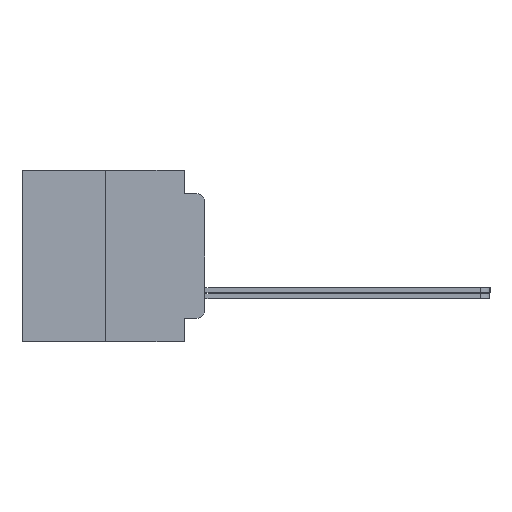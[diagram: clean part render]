
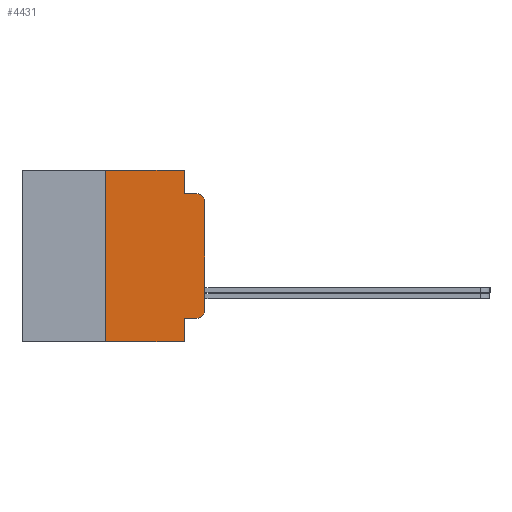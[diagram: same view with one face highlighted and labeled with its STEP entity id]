
A CAD part, left-side view. The second image highlights one B-rep face of the part: STEP entity #4431.
In plain terms, the highlighted planar face has unit normal (-1, 0, 0).
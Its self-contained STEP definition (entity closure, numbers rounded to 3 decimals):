
#132 = VECTOR ( 'NONE', #7905, 1000. ) ;
#256 = DIRECTION ( 'NONE',  ( -1., 0., 0. ) ) ;
#378 = CARTESIAN_POINT ( 'NONE',  ( -75.603, 6.35, -5.486 ) ) ;
#1163 = PLANE ( 'NONE',  #27982 ) ;
#1304 = EDGE_CURVE ( 'NONE', #25499, #4151, #22704, .T. ) ;
#1706 = DIRECTION ( 'NONE',  ( 0., 0., -1. ) ) ;
#2523 = CARTESIAN_POINT ( 'NONE',  ( -75.603, 0.508, -3.975 ) ) ;
#2753 = CARTESIAN_POINT ( 'NONE',  ( -75.603, 1.295, 3.975 ) ) ;
#2827 = CARTESIAN_POINT ( 'NONE',  ( -75.603, 0., -3.467 ) ) ;
#2840 = CIRCLE ( 'NONE', #26638, 0.508 ) ;
#3212 = DIRECTION ( 'NONE',  ( 0., 0., -1. ) ) ;
#3895 = CARTESIAN_POINT ( 'NONE',  ( -75.603, 1.295, 5.486 ) ) ;
#4070 = ORIENTED_EDGE ( 'NONE', *, *, #7823, .F. ) ;
#4151 = VERTEX_POINT ( 'NONE', #2523 ) ;
#4431 = ADVANCED_FACE ( 'NONE', ( #4550 ), #1163, .F. ) ;
#4481 = CARTESIAN_POINT ( 'NONE',  ( -75.603, 1.295, 0. ) ) ;
#4550 = FACE_OUTER_BOUND ( 'NONE', #16458, .T. ) ;
#4566 = VERTEX_POINT ( 'NONE', #24380 ) ;
#4567 = EDGE_CURVE ( 'NONE', #25499, #4566, #9770, .T. ) ;
#5145 = ORIENTED_EDGE ( 'NONE', *, *, #4567, .F. ) ;
#5813 = DIRECTION ( 'NONE',  ( 0., 0., -1. ) ) ;
#5853 = DIRECTION ( 'NONE',  ( 0., 0., -1. ) ) ;
#6031 = LINE ( 'NONE', #15379, #25827 ) ;
#6654 = DIRECTION ( 'NONE',  ( 0., -1., 0. ) ) ;
#6815 = VERTEX_POINT ( 'NONE', #9495 ) ;
#7102 = CARTESIAN_POINT ( 'NONE',  ( -75.603, 0.508, -3.467 ) ) ;
#7295 = ORIENTED_EDGE ( 'NONE', *, *, #21689, .T. ) ;
#7429 = CARTESIAN_POINT ( 'NONE',  ( -75.603, 0., 3.467 ) ) ;
#7537 = EDGE_CURVE ( 'NONE', #4151, #10115, #28331, .T. ) ;
#7823 = EDGE_CURVE ( 'NONE', #12068, #6815, #17882, .T. ) ;
#7905 = DIRECTION ( 'NONE',  ( 0., -1., 0. ) ) ;
#8957 = CARTESIAN_POINT ( 'NONE',  ( -75.603, 0., 5.486 ) ) ;
#9137 = ORIENTED_EDGE ( 'NONE', *, *, #26691, .F. ) ;
#9352 = DIRECTION ( 'NONE',  ( 0., -1., 0. ) ) ;
#9495 = CARTESIAN_POINT ( 'NONE',  ( -75.603, 0.508, 3.975 ) ) ;
#9770 = LINE ( 'NONE', #4481, #10149 ) ;
#9790 = ORIENTED_EDGE ( 'NONE', *, *, #1304, .T. ) ;
#10115 = VERTEX_POINT ( 'NONE', #2827 ) ;
#10149 = VECTOR ( 'NONE', #13047, 1000. ) ;
#11171 = EDGE_CURVE ( 'NONE', #13454, #24006, #14789, .T. ) ;
#11387 = CARTESIAN_POINT ( 'NONE',  ( -75.603, 11.684, 5.486 ) ) ;
#11500 = AXIS2_PLACEMENT_3D ( 'NONE', #7102, #256, #1706 ) ;
#12068 = VERTEX_POINT ( 'NONE', #15317 ) ;
#12388 = VECTOR ( 'NONE', #18362, 1000. ) ;
#13047 = DIRECTION ( 'NONE',  ( 0., 0., -1. ) ) ;
#13218 = EDGE_CURVE ( 'NONE', #27890, #6815, #2840, .T. ) ;
#13454 = VERTEX_POINT ( 'NONE', #19078 ) ;
#13497 = DIRECTION ( 'NONE',  ( 0., 0., 1. ) ) ;
#13861 = CARTESIAN_POINT ( 'NONE',  ( -75.603, 1.295, -3.975 ) ) ;
#14388 = DIRECTION ( 'NONE',  ( -1., 0., 0. ) ) ;
#14654 = ORIENTED_EDGE ( 'NONE', *, *, #23610, .T. ) ;
#14789 = LINE ( 'NONE', #11387, #12388 ) ;
#15317 = CARTESIAN_POINT ( 'NONE',  ( -75.603, 1.295, 3.975 ) ) ;
#15379 = CARTESIAN_POINT ( 'NONE',  ( -75.603, 11.684, -5.486 ) ) ;
#15597 = VECTOR ( 'NONE', #3212, 1000. ) ;
#15895 = DIRECTION ( 'NONE',  ( 0., 0., 1. ) ) ;
#16458 = EDGE_LOOP ( 'NONE', ( #9790, #23973, #7295, #22887, #4070, #9137, #19512, #26929, #14654, #5145 ) ) ;
#16563 = CARTESIAN_POINT ( 'NONE',  ( -75.603, 11.684, 5.486 ) ) ;
#17685 = LINE ( 'NONE', #18348, #15597 ) ;
#17882 = LINE ( 'NONE', #2753, #23119 ) ;
#17950 = LINE ( 'NONE', #8957, #28373 ) ;
#18348 = CARTESIAN_POINT ( 'NONE',  ( -75.603, 1.295, 0. ) ) ;
#18362 = DIRECTION ( 'NONE',  ( 0., -1., 0. ) ) ;
#19078 = CARTESIAN_POINT ( 'NONE',  ( -75.603, 6.35, 5.486 ) ) ;
#19512 = ORIENTED_EDGE ( 'NONE', *, *, #11171, .F. ) ;
#19849 = EDGE_CURVE ( 'NONE', #20235, #13454, #23113, .T. ) ;
#20235 = VERTEX_POINT ( 'NONE', #28207 ) ;
#21007 = VECTOR ( 'NONE', #15895, 1000. ) ;
#21689 = EDGE_CURVE ( 'NONE', #10115, #27890, #17950, .T. ) ;
#22704 = LINE ( 'NONE', #23116, #132 ) ;
#22887 = ORIENTED_EDGE ( 'NONE', *, *, #13218, .T. ) ;
#23113 = LINE ( 'NONE', #378, #21007 ) ;
#23116 = CARTESIAN_POINT ( 'NONE',  ( -75.603, 1.295, -3.975 ) ) ;
#23119 = VECTOR ( 'NONE', #9352, 1000. ) ;
#23280 = DIRECTION ( 'NONE',  ( 1., 0., 0. ) ) ;
#23610 = EDGE_CURVE ( 'NONE', #20235, #4566, #6031, .T. ) ;
#23973 = ORIENTED_EDGE ( 'NONE', *, *, #7537, .T. ) ;
#24006 = VERTEX_POINT ( 'NONE', #3895 ) ;
#24380 = CARTESIAN_POINT ( 'NONE',  ( -75.603, 1.295, -5.486 ) ) ;
#25460 = CARTESIAN_POINT ( 'NONE',  ( -75.603, 0.508, 3.467 ) ) ;
#25499 = VERTEX_POINT ( 'NONE', #13861 ) ;
#25827 = VECTOR ( 'NONE', #6654, 1000. ) ;
#26638 = AXIS2_PLACEMENT_3D ( 'NONE', #25460, #14388, #5853 ) ;
#26691 = EDGE_CURVE ( 'NONE', #24006, #12068, #17685, .T. ) ;
#26929 = ORIENTED_EDGE ( 'NONE', *, *, #19849, .F. ) ;
#27890 = VERTEX_POINT ( 'NONE', #7429 ) ;
#27982 = AXIS2_PLACEMENT_3D ( 'NONE', #16563, #23280, #5813 ) ;
#28207 = CARTESIAN_POINT ( 'NONE',  ( -75.603, 6.35, -5.486 ) ) ;
#28331 = CIRCLE ( 'NONE', #11500, 0.508 ) ;
#28373 = VECTOR ( 'NONE', #13497, 1000. ) ;
